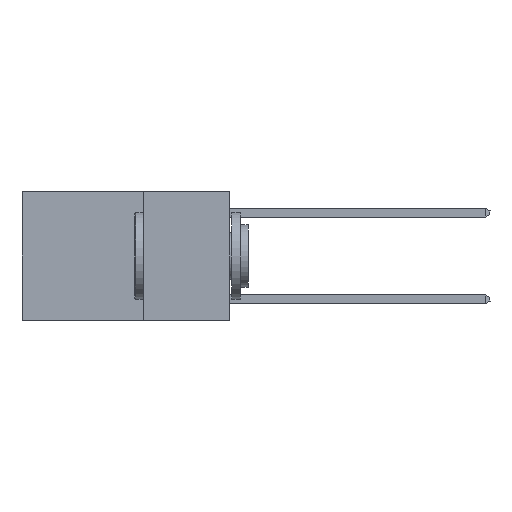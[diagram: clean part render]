
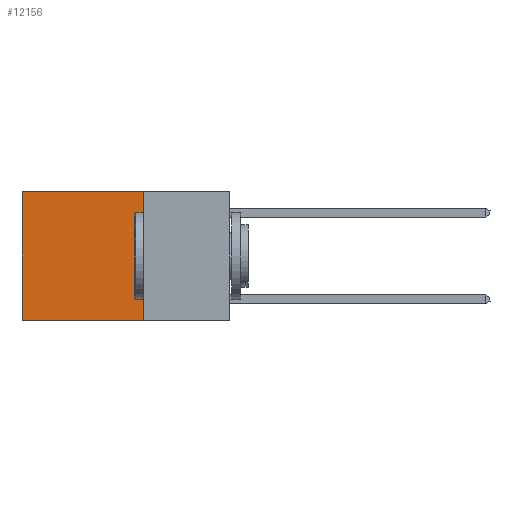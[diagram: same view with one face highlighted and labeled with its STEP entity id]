
A CAD part, left-side view. The second image highlights one B-rep face of the part: STEP entity #12156.
In plain terms, the highlighted planar face has unit normal (-1, 0, 0).
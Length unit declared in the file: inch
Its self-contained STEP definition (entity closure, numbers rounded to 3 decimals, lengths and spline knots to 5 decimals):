
#81 = ORIENTED_EDGE ( 'NONE', *, *, #12414, .F. ) ;
#919 = ORIENTED_EDGE ( 'NONE', *, *, #6110, .T. ) ;
#1546 = CARTESIAN_POINT ( 'NONE',  ( 0.2625, 0.25, 0. ) ) ;
#2846 = FACE_OUTER_BOUND ( 'NONE', #3000, .T. ) ;
#3000 = EDGE_LOOP ( 'NONE', ( #919, #81, #5132, #7599 ) ) ;
#3031 = DIRECTION ( 'NONE',  ( 0., 0., -1. ) ) ;
#3473 = AXIS2_PLACEMENT_3D ( 'NONE', #1546, #12046, #18210 ) ;
#3632 = LINE ( 'NONE', #15815, #12441 ) ;
#4037 = VERTEX_POINT ( 'NONE', #9137 ) ;
#5132 = ORIENTED_EDGE ( 'NONE', *, *, #14650, .F. ) ;
#5665 = CARTESIAN_POINT ( 'NONE',  ( 0.2625, 0.25, -0.37 ) ) ;
#6110 = EDGE_CURVE ( 'NONE', #6135, #4037, #9634, .T. ) ;
#6135 = VERTEX_POINT ( 'NONE', #6834 ) ;
#6834 = CARTESIAN_POINT ( 'NONE',  ( 0.2625, 0.6, 0. ) ) ;
#7554 = CARTESIAN_POINT ( 'NONE',  ( 0.2625, 0.25, 0. ) ) ;
#7599 = ORIENTED_EDGE ( 'NONE', *, *, #17678, .T. ) ;
#7885 = CARTESIAN_POINT ( 'NONE',  ( 0.2625, 0.25, 0. ) ) ;
#9137 = CARTESIAN_POINT ( 'NONE',  ( 0.2625, 0.6, -0.37 ) ) ;
#9634 = LINE ( 'NONE', #10841, #16094 ) ;
#9742 = DIRECTION ( 'NONE',  ( 0., 1., 0. ) ) ;
#10841 = CARTESIAN_POINT ( 'NONE',  ( 0.2625, 0.6, 0. ) ) ;
#11267 = VERTEX_POINT ( 'NONE', #7885 ) ;
#11812 = VECTOR ( 'NONE', #3031, 39.37008 ) ;
#12046 = DIRECTION ( 'NONE',  ( 1., 0., 0. ) ) ;
#12156 = ADVANCED_FACE ( 'NONE', ( #2846 ), #15233, .F. ) ;
#12414 = EDGE_CURVE ( 'NONE', #19023, #4037, #3632, .T. ) ;
#12441 = VECTOR ( 'NONE', #9742, 39.37008 ) ;
#14650 = EDGE_CURVE ( 'NONE', #11267, #19023, #15122, .T. ) ;
#15122 = LINE ( 'NONE', #16709, #11812 ) ;
#15233 = PLANE ( 'NONE',  #3473 ) ;
#15815 = CARTESIAN_POINT ( 'NONE',  ( 0.2625, 0.25, -0.37 ) ) ;
#16094 = VECTOR ( 'NONE', #17102, 39.37008 ) ;
#16433 = DIRECTION ( 'NONE',  ( 0., 1., 0. ) ) ;
#16709 = CARTESIAN_POINT ( 'NONE',  ( 0.2625, 0.25, 0. ) ) ;
#17102 = DIRECTION ( 'NONE',  ( 0., 0., -1. ) ) ;
#17678 = EDGE_CURVE ( 'NONE', #11267, #6135, #19632, .T. ) ;
#18210 = DIRECTION ( 'NONE',  ( 0., 0., -1. ) ) ;
#18391 = VECTOR ( 'NONE', #16433, 39.37008 ) ;
#19023 = VERTEX_POINT ( 'NONE', #5665 ) ;
#19632 = LINE ( 'NONE', #7554, #18391 ) ;
